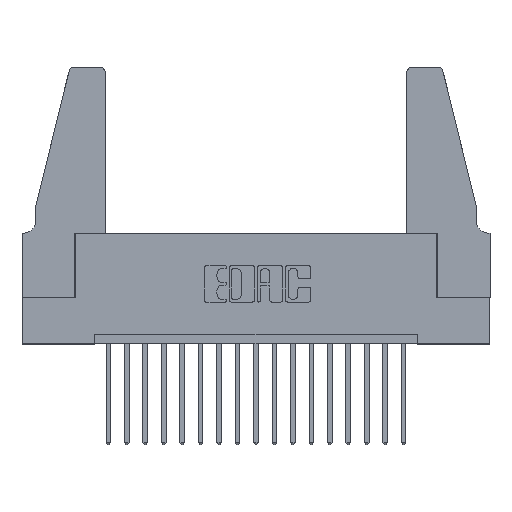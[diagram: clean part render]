
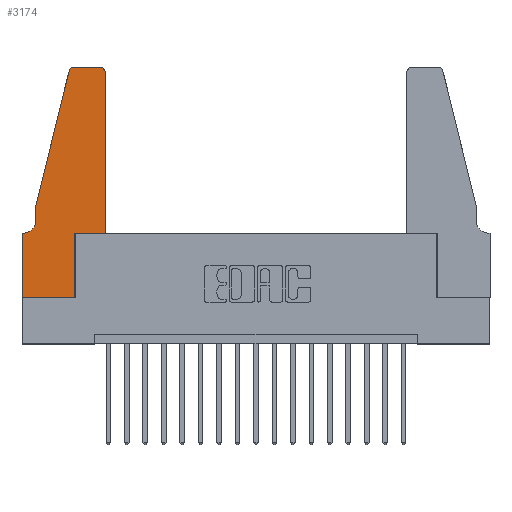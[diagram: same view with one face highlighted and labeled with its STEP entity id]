
A CAD part, top view. The second image highlights one B-rep face of the part: STEP entity #3174.
In plain terms, the highlighted planar face has unit normal (0, 0, 1).
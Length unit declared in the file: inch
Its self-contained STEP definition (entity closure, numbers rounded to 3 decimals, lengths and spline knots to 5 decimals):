
#113 = ORIENTED_EDGE ( 'NONE', *, *, #4411, .T. ) ;
#207 = EDGE_CURVE ( 'NONE', #12516, #14726, #5632, .T. ) ;
#234 = ORIENTED_EDGE ( 'NONE', *, *, #207, .T. ) ;
#373 = FACE_OUTER_BOUND ( 'NONE', #1218, .T. ) ;
#379 = CARTESIAN_POINT ( 'NONE',  ( 0.0055, 0.42, 0.37 ) ) ;
#1218 = EDGE_LOOP ( 'NONE', ( #9526, #234, #113, #16810, #13674, #17167, #15226, #8393, #7453, #3452, #4901, #5936 ) ) ;
#1911 = EDGE_CURVE ( 'NONE', #12417, #10788, #6254, .T. ) ;
#1970 = VECTOR ( 'NONE', #6280, 39.37008 ) ;
#3149 = AXIS2_PLACEMENT_3D ( 'NONE', #17406, #11797, #3316 ) ;
#3174 = ADVANCED_FACE ( 'NONE', ( #373 ), #4618, .T. ) ;
#3285 = VERTEX_POINT ( 'NONE', #17071 ) ;
#3316 = DIRECTION ( 'NONE',  ( 1., 0., 0. ) ) ;
#3373 = DIRECTION ( 'NONE',  ( -1., 0., 0. ) ) ;
#3389 = LINE ( 'NONE', #8405, #7358 ) ;
#3452 = ORIENTED_EDGE ( 'NONE', *, *, #12839, .T. ) ;
#3677 = CARTESIAN_POINT ( 'NONE',  ( 0.2865, 0.35, 0.37 ) ) ;
#3918 = CARTESIAN_POINT ( 'NONE',  ( 0.4205, 1.22, 0.37 ) ) ;
#4411 = EDGE_CURVE ( 'NONE', #14726, #11088, #5199, .T. ) ;
#4434 = EDGE_CURVE ( 'NONE', #16097, #13454, #16516, .T. ) ;
#4618 = PLANE ( 'NONE',  #3149 ) ;
#4825 = CARTESIAN_POINT ( 'NONE',  ( 0.2605, 1.25, 0.37 ) ) ;
#4846 = DIRECTION ( 'NONE',  ( 1., 0., 0. ) ) ;
#4901 = ORIENTED_EDGE ( 'NONE', *, *, #6508, .T. ) ;
#5066 = CARTESIAN_POINT ( 'NONE',  ( 0.0755, 0.5, 0.37 ) ) ;
#5126 = EDGE_CURVE ( 'NONE', #10788, #3285, #10058, .T. ) ;
#5199 = LINE ( 'NONE', #9451, #12983 ) ;
#5632 = CIRCLE ( 'NONE', #6276, 0.03 ) ;
#5637 = CARTESIAN_POINT ( 'NONE',  ( 0.4505, 0.35, 0.37 ) ) ;
#5723 = CIRCLE ( 'NONE', #13229, 0.03 ) ;
#5799 = LINE ( 'NONE', #4825, #10017 ) ;
#5936 = ORIENTED_EDGE ( 'NONE', *, *, #11759, .T. ) ;
#6254 = LINE ( 'NONE', #14179, #11829 ) ;
#6276 = AXIS2_PLACEMENT_3D ( 'NONE', #10610, #9429, #17757 ) ;
#6280 = DIRECTION ( 'NONE',  ( -1., 0., 0. ) ) ;
#6489 = DIRECTION ( 'NONE',  ( 0., -1., 0. ) ) ;
#6508 = EDGE_CURVE ( 'NONE', #14920, #15794, #3389, .T. ) ;
#7077 = CARTESIAN_POINT ( 'NONE',  ( 0.284, 1.25, 0.37 ) ) ;
#7298 = EDGE_CURVE ( 'NONE', #11088, #16097, #13771, .T. ) ;
#7358 = VECTOR ( 'NONE', #15496, 39.37008 ) ;
#7424 = DIRECTION ( 'NONE',  ( -1., 0., 0. ) ) ;
#7453 = ORIENTED_EDGE ( 'NONE', *, *, #12957, .T. ) ;
#7510 = DIRECTION ( 'NONE',  ( -0.239, -0.971, 0. ) ) ;
#7852 = EDGE_CURVE ( 'NONE', #13454, #12417, #17276, .T. ) ;
#8043 = DIRECTION ( 'NONE',  ( 0., 1., 0. ) ) ;
#8393 = ORIENTED_EDGE ( 'NONE', *, *, #5126, .T. ) ;
#8405 = CARTESIAN_POINT ( 'NONE',  ( 0.4505, 0.35, 0.37 ) ) ;
#8507 = DIRECTION ( 'NONE',  ( 0., -1., 0. ) ) ;
#8657 = CARTESIAN_POINT ( 'NONE',  ( 0., 0., 0.37 ) ) ;
#8778 = LINE ( 'NONE', #14583, #14348 ) ;
#9100 = CARTESIAN_POINT ( 'NONE',  ( 0.2865, 0.35, 0.37 ) ) ;
#9132 = CARTESIAN_POINT ( 'NONE',  ( 0.0055, 0.35, 0.37 ) ) ;
#9429 = DIRECTION ( 'NONE',  ( 0., 0., 1. ) ) ;
#9451 = CARTESIAN_POINT ( 'NONE',  ( 0.0755, 0.5, 0.37 ) ) ;
#9526 = ORIENTED_EDGE ( 'NONE', *, *, #9638, .T. ) ;
#9638 = EDGE_CURVE ( 'NONE', #10444, #12516, #5799, .T. ) ;
#9670 = DIRECTION ( 'NONE',  ( 1., 0., 0. ) ) ;
#9870 = CARTESIAN_POINT ( 'NONE',  ( 0., 0.35, 0.37 ) ) ;
#10017 = VECTOR ( 'NONE', #7424, 39.37008 ) ;
#10058 = LINE ( 'NONE', #14020, #17134 ) ;
#10368 = DIRECTION ( 'NONE',  ( 0., 0., -1. ) ) ;
#10444 = VERTEX_POINT ( 'NONE', #16957 ) ;
#10610 = CARTESIAN_POINT ( 'NONE',  ( 0.284, 1.22, 0.37 ) ) ;
#10788 = VERTEX_POINT ( 'NONE', #8657 ) ;
#11088 = VERTEX_POINT ( 'NONE', #17536 ) ;
#11648 = CARTESIAN_POINT ( 'NONE',  ( 0.0755, 0.42, 0.37 ) ) ;
#11672 = VECTOR ( 'NONE', #8043, 39.37008 ) ;
#11752 = CARTESIAN_POINT ( 'NONE',  ( 0.0755, 0.35, 0.37 ) ) ;
#11759 = EDGE_CURVE ( 'NONE', #15794, #10444, #5723, .T. ) ;
#11797 = DIRECTION ( 'NONE',  ( 0., 0., 1. ) ) ;
#11829 = VECTOR ( 'NONE', #8507, 39.37008 ) ;
#12417 = VERTEX_POINT ( 'NONE', #9870 ) ;
#12516 = VERTEX_POINT ( 'NONE', #7077 ) ;
#12826 = VERTEX_POINT ( 'NONE', #9100 ) ;
#12839 = EDGE_CURVE ( 'NONE', #12826, #14920, #8778, .T. ) ;
#12957 = EDGE_CURVE ( 'NONE', #3285, #12826, #15434, .T. ) ;
#12983 = VECTOR ( 'NONE', #7510, 39.37008 ) ;
#13229 = AXIS2_PLACEMENT_3D ( 'NONE', #3918, #15232, #16485 ) ;
#13249 = AXIS2_PLACEMENT_3D ( 'NONE', #379, #10368, #3373 ) ;
#13329 = VECTOR ( 'NONE', #6489, 39.37008 ) ;
#13454 = VERTEX_POINT ( 'NONE', #9132 ) ;
#13674 = ORIENTED_EDGE ( 'NONE', *, *, #4434, .T. ) ;
#13771 = LINE ( 'NONE', #5066, #13329 ) ;
#14020 = CARTESIAN_POINT ( 'NONE',  ( 0., 0., 0.37 ) ) ;
#14179 = CARTESIAN_POINT ( 'NONE',  ( 0., 0., 0.37 ) ) ;
#14348 = VECTOR ( 'NONE', #4846, 39.37008 ) ;
#14583 = CARTESIAN_POINT ( 'NONE',  ( 0.4505, 0.35, 0.37 ) ) ;
#14726 = VERTEX_POINT ( 'NONE', #15020 ) ;
#14920 = VERTEX_POINT ( 'NONE', #5637 ) ;
#15020 = CARTESIAN_POINT ( 'NONE',  ( 0.25487, 1.22718, 0.37 ) ) ;
#15226 = ORIENTED_EDGE ( 'NONE', *, *, #1911, .T. ) ;
#15232 = DIRECTION ( 'NONE',  ( 0., 0., 1. ) ) ;
#15434 = LINE ( 'NONE', #3677, #11672 ) ;
#15496 = DIRECTION ( 'NONE',  ( 0., 1., 0. ) ) ;
#15570 = CARTESIAN_POINT ( 'NONE',  ( 0.4505, 1.22, 0.37 ) ) ;
#15794 = VERTEX_POINT ( 'NONE', #15570 ) ;
#16097 = VERTEX_POINT ( 'NONE', #11648 ) ;
#16485 = DIRECTION ( 'NONE',  ( 1., 0., 0. ) ) ;
#16516 = CIRCLE ( 'NONE', #13249, 0.07 ) ;
#16810 = ORIENTED_EDGE ( 'NONE', *, *, #7298, .T. ) ;
#16957 = CARTESIAN_POINT ( 'NONE',  ( 0.4205, 1.25, 0.37 ) ) ;
#17071 = CARTESIAN_POINT ( 'NONE',  ( 0.2865, 0., 0.37 ) ) ;
#17134 = VECTOR ( 'NONE', #9670, 39.37008 ) ;
#17167 = ORIENTED_EDGE ( 'NONE', *, *, #7852, .T. ) ;
#17276 = LINE ( 'NONE', #11752, #1970 ) ;
#17406 = CARTESIAN_POINT ( 'NONE',  ( 0., 0.35, 0.37 ) ) ;
#17536 = CARTESIAN_POINT ( 'NONE',  ( 0.0755, 0.5, 0.37 ) ) ;
#17757 = DIRECTION ( 'NONE',  ( 1., 0., 0. ) ) ;
